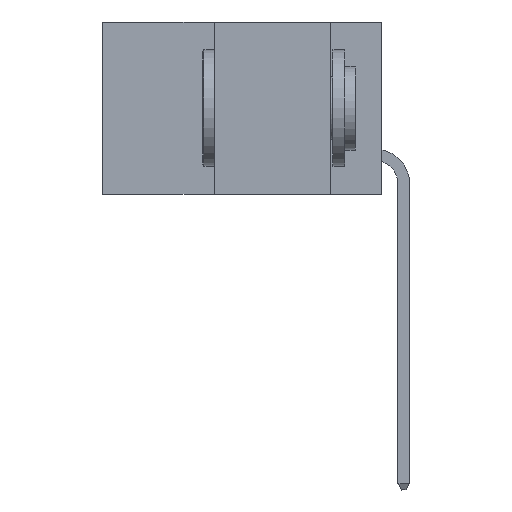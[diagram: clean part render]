
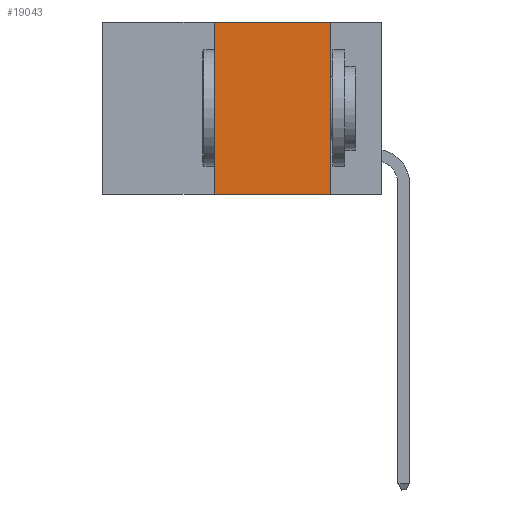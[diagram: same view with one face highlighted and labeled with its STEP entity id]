
A CAD part, left-side view. The second image highlights one B-rep face of the part: STEP entity #19043.
In plain terms, the highlighted planar face has unit normal (-1, 0, 0).
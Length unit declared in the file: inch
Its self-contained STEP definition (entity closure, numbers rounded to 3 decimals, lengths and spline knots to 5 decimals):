
#487 = DIRECTION ( 'NONE',  ( 0., -1., 0. ) ) ;
#1359 = EDGE_CURVE ( 'NONE', #28439, #7071, #12534, .T. ) ;
#2051 = VECTOR ( 'NONE', #24664, 39.37008 ) ;
#2192 = DIRECTION ( 'NONE',  ( 1., 0., 0. ) ) ;
#2724 = CARTESIAN_POINT ( 'NONE',  ( 0., 0.6, 0. ) ) ;
#4344 = CARTESIAN_POINT ( 'NONE',  ( 0., 0.6, 0. ) ) ;
#4644 = PLANE ( 'NONE',  #19705 ) ;
#4803 = VECTOR ( 'NONE', #17342, 39.37008 ) ;
#5726 = ORIENTED_EDGE ( 'NONE', *, *, #6382, .F. ) ;
#6194 = CARTESIAN_POINT ( 'NONE',  ( 0., 0.36, -0.37 ) ) ;
#6382 = EDGE_CURVE ( 'NONE', #23550, #16304, #10649, .T. ) ;
#6454 = ORIENTED_EDGE ( 'NONE', *, *, #1359, .F. ) ;
#7071 = VERTEX_POINT ( 'NONE', #10785 ) ;
#8502 = CARTESIAN_POINT ( 'NONE',  ( 0., 0.36, 0. ) ) ;
#8520 = CARTESIAN_POINT ( 'NONE',  ( 0., 0.11, -0.37 ) ) ;
#8755 = CARTESIAN_POINT ( 'NONE',  ( 0., 0.11, 0. ) ) ;
#10649 = LINE ( 'NONE', #8755, #20785 ) ;
#10785 = CARTESIAN_POINT ( 'NONE',  ( 0., 0.36, 0. ) ) ;
#12534 = LINE ( 'NONE', #8502, #2051 ) ;
#15715 = ORIENTED_EDGE ( 'NONE', *, *, #24323, .T. ) ;
#15721 = LINE ( 'NONE', #2724, #23638 ) ;
#16304 = VERTEX_POINT ( 'NONE', #8520 ) ;
#16429 = FACE_OUTER_BOUND ( 'NONE', #28143, .T. ) ;
#17109 = DIRECTION ( 'NONE',  ( 0., 0., -1. ) ) ;
#17342 = DIRECTION ( 'NONE',  ( 0., -1., 0. ) ) ;
#19043 = ADVANCED_FACE ( 'NONE', ( #16429 ), #4644, .F. ) ;
#19638 = EDGE_CURVE ( 'NONE', #7071, #23550, #15721, .T. ) ;
#19682 = CARTESIAN_POINT ( 'NONE',  ( 0., 0.6, -0.37 ) ) ;
#19705 = AXIS2_PLACEMENT_3D ( 'NONE', #4344, #2192, #17109 ) ;
#20754 = ORIENTED_EDGE ( 'NONE', *, *, #19638, .F. ) ;
#20758 = LINE ( 'NONE', #19682, #4803 ) ;
#20785 = VECTOR ( 'NONE', #27179, 39.37008 ) ;
#23550 = VERTEX_POINT ( 'NONE', #23837 ) ;
#23638 = VECTOR ( 'NONE', #487, 39.37008 ) ;
#23837 = CARTESIAN_POINT ( 'NONE',  ( 0., 0.11, 0. ) ) ;
#24323 = EDGE_CURVE ( 'NONE', #28439, #16304, #20758, .T. ) ;
#24664 = DIRECTION ( 'NONE',  ( 0., 0., 1. ) ) ;
#27179 = DIRECTION ( 'NONE',  ( 0., 0., -1. ) ) ;
#28143 = EDGE_LOOP ( 'NONE', ( #5726, #20754, #6454, #15715 ) ) ;
#28439 = VERTEX_POINT ( 'NONE', #6194 ) ;
